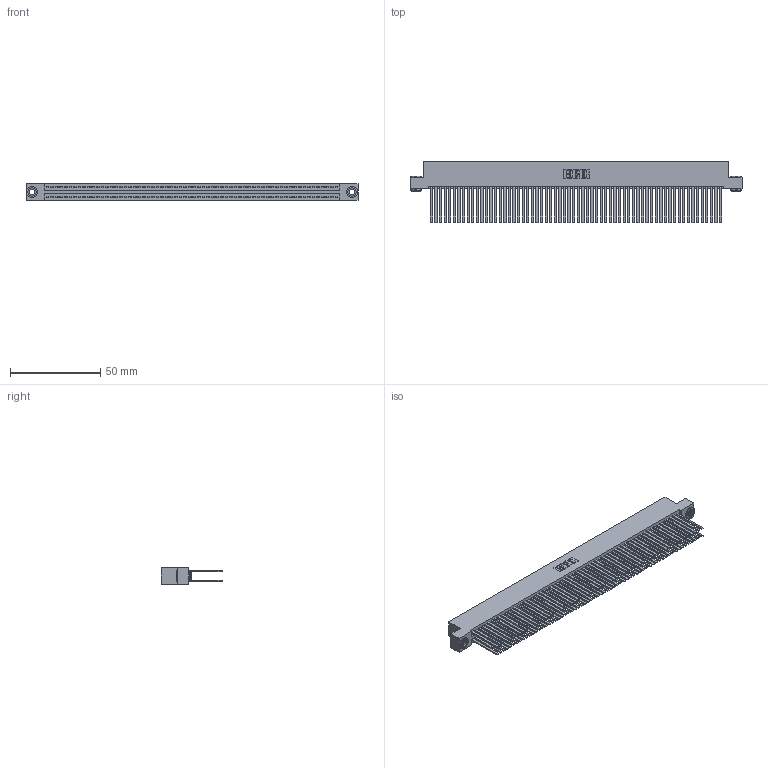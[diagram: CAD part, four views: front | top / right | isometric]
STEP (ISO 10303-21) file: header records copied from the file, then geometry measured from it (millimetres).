
FILE_DESCRIPTION (( 'STEP AP203' ), '1' );
FILE_NAME ('345-128-544-203.STEP', '2018-10-19T20:50:41', ( '' ), ( '' ), 'SwSTEP 2.0', 'SolidWorks 2016', '' );
FILE_SCHEMA (( 'CONFIG_CONTROL_DESIGN' ));
Length unit declared in the file: inch
Products named in the file (4): 345-250-002_345-250-002-102; 345-292-001_345-293-144; 345 Part_Flush Mounting Lugs - 0.156 Dia-TH; 345-128-544-203
Assembly tree (131 placements, depth 2):
  345-128-544-203
    345 Part_Flush Mounting Lugs - 0.156 Dia-TH
    345-292-001_345-293-144  x128
    345-250-002_345-250-002-102  x2
Bounding box: 183.77 x 33.96 x 9.4 mm (x, y, z)
Volume: 19869.4 mm3; surface area: 35260.4 mm2
Topology: 131 solids, 131 shells, 5796 faces, 17185 edges, 11282 vertices
Faces by surface type: plane 3802, cylinder 1986, cone 8
Entity records: 47720 total; most frequent: CARTESIAN_POINT 7951, ORIENTED_EDGE 7878, DIRECTION 7013, EDGE_CURVE 3939, LINE 3531, VECTOR 3531, VERTEX_POINT 2622, AXIS2_PLACEMENT_3D 1741
